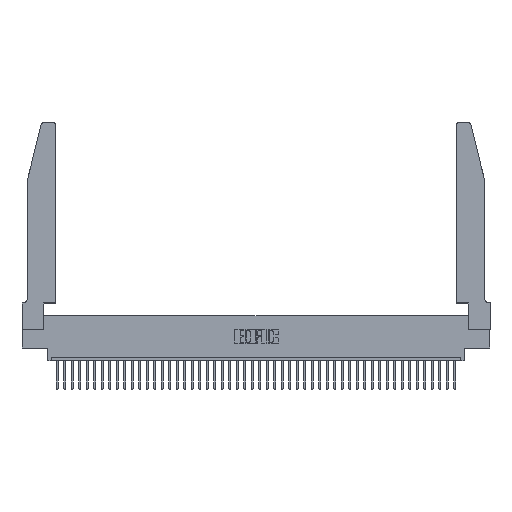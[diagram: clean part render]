
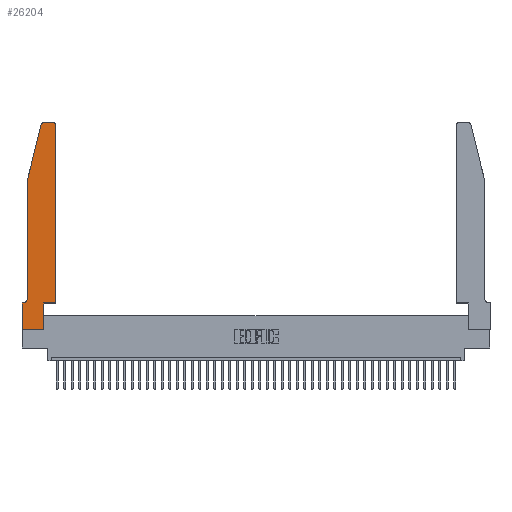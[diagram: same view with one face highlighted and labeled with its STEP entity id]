
A CAD part, top view. The second image highlights one B-rep face of the part: STEP entity #26204.
In plain terms, the highlighted planar face has unit normal (0, 0, 1).
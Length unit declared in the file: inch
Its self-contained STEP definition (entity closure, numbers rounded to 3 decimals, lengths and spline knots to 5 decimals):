
#188 = DIRECTION ( 'NONE',  ( 0., 0., 1. ) ) ;
#1225 = CARTESIAN_POINT ( 'NONE',  ( 0.25487, 2.72718, 0.37 ) ) ;
#1463 = VERTEX_POINT ( 'NONE', #24472 ) ;
#1967 = CARTESIAN_POINT ( 'NONE',  ( 0.0755, 0.42, 0.37 ) ) ;
#2710 = ORIENTED_EDGE ( 'NONE', *, *, #37840, .T. ) ;
#2808 = DIRECTION ( 'NONE',  ( 0., 0., -1. ) ) ;
#4865 = CARTESIAN_POINT ( 'NONE',  ( 0.4505, 0.35, 0.37 ) ) ;
#5183 = LINE ( 'NONE', #22936, #8925 ) ;
#5929 = LINE ( 'NONE', #41716, #29305 ) ;
#5959 = CARTESIAN_POINT ( 'NONE',  ( 0.4505, 0.35, 0.37 ) ) ;
#6237 = DIRECTION ( 'NONE',  ( 0., 1., 0. ) ) ;
#6407 = VECTOR ( 'NONE', #10090, 39.37008 ) ;
#6655 = CARTESIAN_POINT ( 'NONE',  ( 0.2605, 2.75, 0.37 ) ) ;
#7117 = AXIS2_PLACEMENT_3D ( 'NONE', #25814, #32761, #15703 ) ;
#7665 = CARTESIAN_POINT ( 'NONE',  ( 0.4205, 2.75, 0.37 ) ) ;
#7754 = CARTESIAN_POINT ( 'NONE',  ( 0.2865, 0.35, 0.37 ) ) ;
#7978 = VECTOR ( 'NONE', #17842, 39.37008 ) ;
#8252 = EDGE_CURVE ( 'NONE', #32440, #38769, #10275, .T. ) ;
#8261 = VERTEX_POINT ( 'NONE', #34957 ) ;
#8597 = DIRECTION ( 'NONE',  ( 0., 1., 0. ) ) ;
#8717 = ORIENTED_EDGE ( 'NONE', *, *, #28906, .T. ) ;
#8866 = AXIS2_PLACEMENT_3D ( 'NONE', #13709, #188, #14112 ) ;
#8925 = VECTOR ( 'NONE', #29861, 39.37008 ) ;
#9085 = EDGE_CURVE ( 'NONE', #17066, #8261, #5929, .T. ) ;
#9111 = ORIENTED_EDGE ( 'NONE', *, *, #22099, .T. ) ;
#9362 = CARTESIAN_POINT ( 'NONE',  ( 0.2865, 0.35, 0.37 ) ) ;
#10090 = DIRECTION ( 'NONE',  ( -1., 0., 0. ) ) ;
#10183 = CARTESIAN_POINT ( 'NONE',  ( 0.0755, 2., 0.37 ) ) ;
#10275 = LINE ( 'NONE', #4865, #27782 ) ;
#10433 = VECTOR ( 'NONE', #6237, 39.37008 ) ;
#11803 = LINE ( 'NONE', #5959, #31360 ) ;
#12610 = AXIS2_PLACEMENT_3D ( 'NONE', #26704, #2808, #26546 ) ;
#12942 = CARTESIAN_POINT ( 'NONE',  ( 0.4205, 2.72, 0.37 ) ) ;
#13709 = CARTESIAN_POINT ( 'NONE',  ( 0.284, 2.72, 0.37 ) ) ;
#13806 = CIRCLE ( 'NONE', #12610, 0.07 ) ;
#13822 = LINE ( 'NONE', #6655, #6407 ) ;
#14112 = DIRECTION ( 'NONE',  ( 1., 0., 0. ) ) ;
#14353 = LINE ( 'NONE', #41443, #7978 ) ;
#14524 = DIRECTION ( 'NONE',  ( 0., -1., 0. ) ) ;
#15361 = CIRCLE ( 'NONE', #8866, 0.03 ) ;
#15381 = ORIENTED_EDGE ( 'NONE', *, *, #31071, .T. ) ;
#15694 = CARTESIAN_POINT ( 'NONE',  ( 0.4505, 2.72, 0.37 ) ) ;
#15703 = DIRECTION ( 'NONE',  ( 1., 0., 0. ) ) ;
#16000 = PLANE ( 'NONE',  #7117 ) ;
#16159 = CARTESIAN_POINT ( 'NONE',  ( 0.284, 2.75, 0.37 ) ) ;
#16307 = ORIENTED_EDGE ( 'NONE', *, *, #41543, .T. ) ;
#16797 = CARTESIAN_POINT ( 'NONE',  ( 0.0755, 2., 0.37 ) ) ;
#17066 = VERTEX_POINT ( 'NONE', #40248 ) ;
#17842 = DIRECTION ( 'NONE',  ( -1., 0., 0. ) ) ;
#18284 = ORIENTED_EDGE ( 'NONE', *, *, #33989, .T. ) ;
#18563 = EDGE_CURVE ( 'NONE', #38162, #1463, #13806, .T. ) ;
#18691 = ORIENTED_EDGE ( 'NONE', *, *, #32600, .T. ) ;
#19467 = EDGE_LOOP ( 'NONE', ( #21997, #2710, #18284, #29626, #40531, #18691, #28075, #16307, #8717, #15381, #23281, #9111 ) ) ;
#19754 = FACE_OUTER_BOUND ( 'NONE', #19467, .T. ) ;
#20125 = DIRECTION ( 'NONE',  ( 0., -1., 0. ) ) ;
#20407 = AXIS2_PLACEMENT_3D ( 'NONE', #12942, #26721, #23184 ) ;
#21997 = ORIENTED_EDGE ( 'NONE', *, *, #37286, .T. ) ;
#22099 = EDGE_CURVE ( 'NONE', #38769, #22656, #22231, .T. ) ;
#22231 = CIRCLE ( 'NONE', #20407, 0.03 ) ;
#22656 = VERTEX_POINT ( 'NONE', #7665 ) ;
#22936 = CARTESIAN_POINT ( 'NONE',  ( 0.0755, 2., 0.37 ) ) ;
#23184 = DIRECTION ( 'NONE',  ( 1., 0., 0. ) ) ;
#23281 = ORIENTED_EDGE ( 'NONE', *, *, #8252, .T. ) ;
#24472 = CARTESIAN_POINT ( 'NONE',  ( 0.0055, 0.35, 0.37 ) ) ;
#24939 = VECTOR ( 'NONE', #20125, 39.37008 ) ;
#25365 = VERTEX_POINT ( 'NONE', #16159 ) ;
#25465 = LINE ( 'NONE', #10183, #24939 ) ;
#25497 = DIRECTION ( 'NONE',  ( 1., 0., 0. ) ) ;
#25814 = CARTESIAN_POINT ( 'NONE',  ( 0., 0.35, 0.37 ) ) ;
#25903 = CARTESIAN_POINT ( 'NONE',  ( 0.2865, 0., 0.37 ) ) ;
#26204 = ADVANCED_FACE ( 'NONE', ( #19754 ), #16000, .T. ) ;
#26546 = DIRECTION ( 'NONE',  ( -1., 0., 0. ) ) ;
#26704 = CARTESIAN_POINT ( 'NONE',  ( 0.0055, 0.42, 0.37 ) ) ;
#26721 = DIRECTION ( 'NONE',  ( 0., 0., 1. ) ) ;
#27782 = VECTOR ( 'NONE', #8597, 39.37008 ) ;
#28075 = ORIENTED_EDGE ( 'NONE', *, *, #9085, .T. ) ;
#28472 = LINE ( 'NONE', #9362, #10433 ) ;
#28906 = EDGE_CURVE ( 'NONE', #39659, #43164, #28472, .T. ) ;
#29305 = VECTOR ( 'NONE', #14524, 39.37008 ) ;
#29626 = ORIENTED_EDGE ( 'NONE', *, *, #37640, .T. ) ;
#29861 = DIRECTION ( 'NONE',  ( -0.239, -0.971, 0. ) ) ;
#31071 = EDGE_CURVE ( 'NONE', #43164, #32440, #11803, .T. ) ;
#31360 = VECTOR ( 'NONE', #32951, 39.37008 ) ;
#32440 = VERTEX_POINT ( 'NONE', #37180 ) ;
#32600 = EDGE_CURVE ( 'NONE', #1463, #17066, #14353, .T. ) ;
#32761 = DIRECTION ( 'NONE',  ( 0., 0., 1. ) ) ;
#32951 = DIRECTION ( 'NONE',  ( 1., 0., 0. ) ) ;
#33989 = EDGE_CURVE ( 'NONE', #35576, #41198, #5183, .T. ) ;
#34050 = VECTOR ( 'NONE', #25497, 39.37008 ) ;
#34957 = CARTESIAN_POINT ( 'NONE',  ( 0., 0., 0.37 ) ) ;
#35576 = VERTEX_POINT ( 'NONE', #1225 ) ;
#36198 = LINE ( 'NONE', #38525, #34050 ) ;
#37180 = CARTESIAN_POINT ( 'NONE',  ( 0.4505, 0.35, 0.37 ) ) ;
#37286 = EDGE_CURVE ( 'NONE', #22656, #25365, #13822, .T. ) ;
#37640 = EDGE_CURVE ( 'NONE', #41198, #38162, #25465, .T. ) ;
#37840 = EDGE_CURVE ( 'NONE', #25365, #35576, #15361, .T. ) ;
#38162 = VERTEX_POINT ( 'NONE', #1967 ) ;
#38525 = CARTESIAN_POINT ( 'NONE',  ( 0., 0., 0.37 ) ) ;
#38769 = VERTEX_POINT ( 'NONE', #15694 ) ;
#39659 = VERTEX_POINT ( 'NONE', #25903 ) ;
#40248 = CARTESIAN_POINT ( 'NONE',  ( 0., 0.35, 0.37 ) ) ;
#40531 = ORIENTED_EDGE ( 'NONE', *, *, #18563, .T. ) ;
#41198 = VERTEX_POINT ( 'NONE', #16797 ) ;
#41443 = CARTESIAN_POINT ( 'NONE',  ( 0.0755, 0.35, 0.37 ) ) ;
#41543 = EDGE_CURVE ( 'NONE', #8261, #39659, #36198, .T. ) ;
#41716 = CARTESIAN_POINT ( 'NONE',  ( 0., 0., 0.37 ) ) ;
#43164 = VERTEX_POINT ( 'NONE', #7754 ) ;
